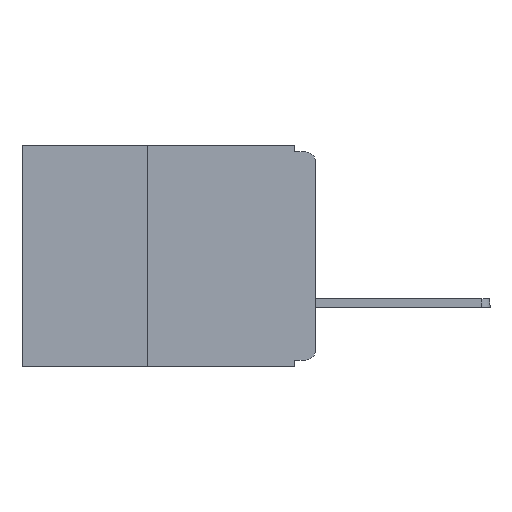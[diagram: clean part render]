
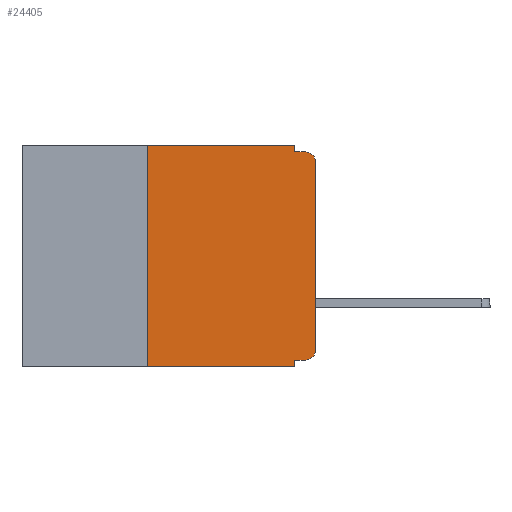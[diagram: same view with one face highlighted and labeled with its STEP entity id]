
A CAD part, left-side view. The second image highlights one B-rep face of the part: STEP entity #24405.
In plain terms, the highlighted planar face has unit normal (-1, 0, 0).
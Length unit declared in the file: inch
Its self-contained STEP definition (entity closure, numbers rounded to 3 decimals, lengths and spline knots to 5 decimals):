
#79 = VERTEX_POINT ( 'NONE', #9024 ) ;
#264 = CARTESIAN_POINT ( 'NONE',  ( 0., 0.031, -0.33 ) ) ;
#451 = CARTESIAN_POINT ( 'NONE',  ( 0., 0.25, 0. ) ) ;
#982 = CARTESIAN_POINT ( 'NONE',  ( 0., 0., 0. ) ) ;
#1054 = DIRECTION ( 'NONE',  ( 0., 0., -1. ) ) ;
#1099 = DIRECTION ( 'NONE',  ( 0., 0., 1. ) ) ;
#1693 = ORIENTED_EDGE ( 'NONE', *, *, #7248, .T. ) ;
#1696 = LINE ( 'NONE', #24039, #24083 ) ;
#1870 = CARTESIAN_POINT ( 'NONE',  ( 0., 0.031, 0. ) ) ;
#1893 = CARTESIAN_POINT ( 'NONE',  ( 0., 0.25, -0.33 ) ) ;
#2077 = EDGE_CURVE ( 'NONE', #79, #8058, #2229, .T. ) ;
#2229 = CIRCLE ( 'NONE', #6597, 0.015 ) ;
#2375 = EDGE_CURVE ( 'NONE', #4968, #21505, #6451, .T. ) ;
#2511 = CARTESIAN_POINT ( 'NONE',  ( 0., 0.031, -0.33 ) ) ;
#3323 = VERTEX_POINT ( 'NONE', #22751 ) ;
#3990 = ORIENTED_EDGE ( 'NONE', *, *, #17459, .T. ) ;
#4032 = LINE ( 'NONE', #20666, #25565 ) ;
#4314 = LINE ( 'NONE', #1870, #13854 ) ;
#4968 = VERTEX_POINT ( 'NONE', #1893 ) ;
#5048 = CARTESIAN_POINT ( 'NONE',  ( 0., 0.031, 0. ) ) ;
#5235 = VECTOR ( 'NONE', #24762, 39.37008 ) ;
#6366 = VERTEX_POINT ( 'NONE', #6734 ) ;
#6451 = LINE ( 'NONE', #24968, #17188 ) ;
#6597 = AXIS2_PLACEMENT_3D ( 'NONE', #20137, #12911, #1054 ) ;
#6734 = CARTESIAN_POINT ( 'NONE',  ( 0., 0.031, -0.01 ) ) ;
#7248 = EDGE_CURVE ( 'NONE', #11842, #79, #9602, .T. ) ;
#7453 = CARTESIAN_POINT ( 'NONE',  ( 0., 0.015, -0.305 ) ) ;
#7788 = EDGE_CURVE ( 'NONE', #4968, #8798, #4032, .T. ) ;
#8049 = DIRECTION ( 'NONE',  ( 1., 0., 0. ) ) ;
#8058 = VERTEX_POINT ( 'NONE', #24724 ) ;
#8692 = ORIENTED_EDGE ( 'NONE', *, *, #2077, .T. ) ;
#8798 = VERTEX_POINT ( 'NONE', #451 ) ;
#9024 = CARTESIAN_POINT ( 'NONE',  ( 0., 0., -0.025 ) ) ;
#9602 = LINE ( 'NONE', #982, #11264 ) ;
#9638 = DIRECTION ( 'NONE',  ( 0., 0., -1. ) ) ;
#9820 = VERTEX_POINT ( 'NONE', #5048 ) ;
#9973 = EDGE_CURVE ( 'NONE', #24876, #3323, #24775, .T. ) ;
#10001 = ORIENTED_EDGE ( 'NONE', *, *, #13568, .F. ) ;
#10129 = CARTESIAN_POINT ( 'NONE',  ( 0., 0.437, 0. ) ) ;
#11264 = VECTOR ( 'NONE', #1099, 39.37008 ) ;
#11723 = AXIS2_PLACEMENT_3D ( 'NONE', #10129, #8049, #23019 ) ;
#11842 = VERTEX_POINT ( 'NONE', #22550 ) ;
#12185 = CARTESIAN_POINT ( 'NONE',  ( 0., 0., -0.32 ) ) ;
#12911 = DIRECTION ( 'NONE',  ( -1., 0., 0. ) ) ;
#13568 = EDGE_CURVE ( 'NONE', #6366, #8058, #1696, .T. ) ;
#13854 = VECTOR ( 'NONE', #27758, 39.37008 ) ;
#14130 = VECTOR ( 'NONE', #24927, 39.37008 ) ;
#14668 = ORIENTED_EDGE ( 'NONE', *, *, #7788, .F. ) ;
#16060 = VECTOR ( 'NONE', #19872, 39.37008 ) ;
#16460 = LINE ( 'NONE', #2511, #16060 ) ;
#17188 = VECTOR ( 'NONE', #22834, 39.37008 ) ;
#17459 = EDGE_CURVE ( 'NONE', #24876, #11842, #18845, .T. ) ;
#17762 = ORIENTED_EDGE ( 'NONE', *, *, #2375, .T. ) ;
#18509 = CARTESIAN_POINT ( 'NONE',  ( 0., 0.015, -0.32 ) ) ;
#18734 = LINE ( 'NONE', #26752, #5235 ) ;
#18845 = CIRCLE ( 'NONE', #23583, 0.015 ) ;
#19872 = DIRECTION ( 'NONE',  ( 0., 0., -1. ) ) ;
#20043 = DIRECTION ( 'NONE',  ( 0., 0., 1. ) ) ;
#20137 = CARTESIAN_POINT ( 'NONE',  ( 0., 0.015, -0.025 ) ) ;
#20139 = EDGE_CURVE ( 'NONE', #9820, #6366, #4314, .T. ) ;
#20666 = CARTESIAN_POINT ( 'NONE',  ( 0., 0.25, -0.33 ) ) ;
#20877 = PLANE ( 'NONE',  #11723 ) ;
#21361 = ORIENTED_EDGE ( 'NONE', *, *, #20139, .F. ) ;
#21505 = VERTEX_POINT ( 'NONE', #264 ) ;
#21506 = EDGE_CURVE ( 'NONE', #3323, #21505, #16460, .T. ) ;
#21825 = ORIENTED_EDGE ( 'NONE', *, *, #21506, .F. ) ;
#21996 = DIRECTION ( 'NONE',  ( 0., -1., 0. ) ) ;
#22434 = DIRECTION ( 'NONE',  ( -1., 0., 0. ) ) ;
#22550 = CARTESIAN_POINT ( 'NONE',  ( 0., 0., -0.305 ) ) ;
#22751 = CARTESIAN_POINT ( 'NONE',  ( 0., 0.031, -0.32 ) ) ;
#22834 = DIRECTION ( 'NONE',  ( 0., -1., 0. ) ) ;
#23019 = DIRECTION ( 'NONE',  ( 0., 0., -1. ) ) ;
#23583 = AXIS2_PLACEMENT_3D ( 'NONE', #7453, #22434, #9638 ) ;
#23840 = ORIENTED_EDGE ( 'NONE', *, *, #24794, .F. ) ;
#24039 = CARTESIAN_POINT ( 'NONE',  ( 0., 0., -0.01 ) ) ;
#24083 = VECTOR ( 'NONE', #21996, 39.37008 ) ;
#24111 = ORIENTED_EDGE ( 'NONE', *, *, #9973, .F. ) ;
#24405 = ADVANCED_FACE ( 'NONE', ( #27322 ), #20877, .F. ) ;
#24724 = CARTESIAN_POINT ( 'NONE',  ( 0., 0.015, -0.01 ) ) ;
#24762 = DIRECTION ( 'NONE',  ( 0., -1., 0. ) ) ;
#24775 = LINE ( 'NONE', #12185, #14130 ) ;
#24794 = EDGE_CURVE ( 'NONE', #8798, #9820, #18734, .T. ) ;
#24876 = VERTEX_POINT ( 'NONE', #18509 ) ;
#24927 = DIRECTION ( 'NONE',  ( 0., 1., 0. ) ) ;
#24968 = CARTESIAN_POINT ( 'NONE',  ( 0., 0.437, -0.33 ) ) ;
#25393 = EDGE_LOOP ( 'NONE', ( #1693, #8692, #10001, #21361, #23840, #14668, #17762, #21825, #24111, #3990 ) ) ;
#25565 = VECTOR ( 'NONE', #20043, 39.37008 ) ;
#26752 = CARTESIAN_POINT ( 'NONE',  ( 0., 0.437, 0. ) ) ;
#27322 = FACE_OUTER_BOUND ( 'NONE', #25393, .T. ) ;
#27758 = DIRECTION ( 'NONE',  ( 0., 0., -1. ) ) ;
